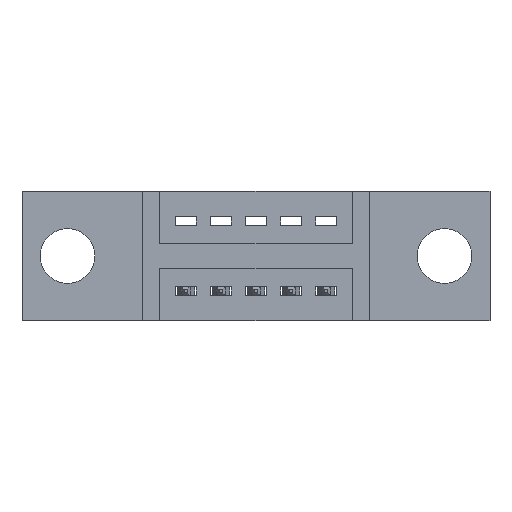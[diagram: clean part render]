
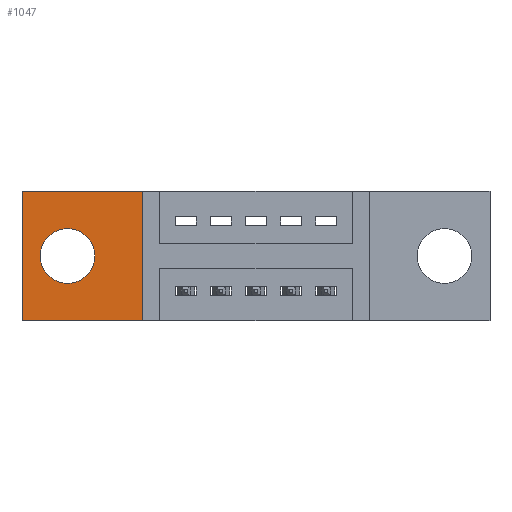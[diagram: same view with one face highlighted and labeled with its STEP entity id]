
A CAD part, front view. The second image highlights one B-rep face of the part: STEP entity #1047.
In plain terms, the highlighted planar face has unit normal (0, -1, 0).
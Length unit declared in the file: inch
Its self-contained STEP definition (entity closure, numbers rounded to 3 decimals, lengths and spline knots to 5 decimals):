
#257 = CIRCLE ( 'NONE', #2262, 0.078 ) ;
#276 = EDGE_CURVE ( 'NONE', #4539, #8290, #7771, .T. ) ;
#394 = VERTEX_POINT ( 'NONE', #4580 ) ;
#573 = FACE_OUTER_BOUND ( 'NONE', #2553, .T. ) ;
#941 = DIRECTION ( 'NONE',  ( -1., 0., 0. ) ) ;
#957 = EDGE_CURVE ( 'NONE', #4929, #394, #257, .T. ) ;
#1047 = ADVANCED_FACE ( 'NONE', ( #6899, #573 ), #6828, .T. ) ;
#1306 = CARTESIAN_POINT ( 'NONE',  ( 0.13, 0.17, -0.185 ) ) ;
#1385 = DIRECTION ( 'NONE',  ( 0., 0., 1. ) ) ;
#1405 = CARTESIAN_POINT ( 'NONE',  ( 0., 0.17, -0.37 ) ) ;
#1478 = CARTESIAN_POINT ( 'NONE',  ( 0., 0.17, 0. ) ) ;
#1729 = DIRECTION ( 'NONE',  ( 1., 0., 0. ) ) ;
#1828 = VERTEX_POINT ( 'NONE', #8216 ) ;
#1973 = CARTESIAN_POINT ( 'NONE',  ( 0., 0.17, 0. ) ) ;
#2034 = DIRECTION ( 'NONE',  ( 0., -1., 0. ) ) ;
#2063 = AXIS2_PLACEMENT_3D ( 'NONE', #1306, #2034, #6825 ) ;
#2262 = AXIS2_PLACEMENT_3D ( 'NONE', #8084, #2614, #6683 ) ;
#2553 = EDGE_LOOP ( 'NONE', ( #7649, #8466, #8158, #4340 ) ) ;
#2614 = DIRECTION ( 'NONE',  ( 0., -1., 0. ) ) ;
#2846 = AXIS2_PLACEMENT_3D ( 'NONE', #1405, #3360, #5383 ) ;
#3050 = CARTESIAN_POINT ( 'NONE',  ( 0., 0.17, -0.37 ) ) ;
#3360 = DIRECTION ( 'NONE',  ( 0., -1., 0. ) ) ;
#3417 = CARTESIAN_POINT ( 'NONE',  ( 0., 0.17, 0. ) ) ;
#4239 = VERTEX_POINT ( 'NONE', #5017 ) ;
#4340 = ORIENTED_EDGE ( 'NONE', *, *, #276, .T. ) ;
#4539 = VERTEX_POINT ( 'NONE', #8808 ) ;
#4580 = CARTESIAN_POINT ( 'NONE',  ( 0.13, 0.17, -0.107 ) ) ;
#4612 = EDGE_CURVE ( 'NONE', #394, #4929, #8253, .T. ) ;
#4929 = VERTEX_POINT ( 'NONE', #8529 ) ;
#4957 = VECTOR ( 'NONE', #1729, 39.37008 ) ;
#5017 = CARTESIAN_POINT ( 'NONE',  ( 0., 0.17, -0.37 ) ) ;
#5274 = LINE ( 'NONE', #5481, #8088 ) ;
#5383 = DIRECTION ( 'NONE',  ( 0., 0., -1. ) ) ;
#5434 = DIRECTION ( 'NONE',  ( 0., 0., -1. ) ) ;
#5479 = LINE ( 'NONE', #1973, #7528 ) ;
#5481 = CARTESIAN_POINT ( 'NONE',  ( 0.3425, 0.17, 0. ) ) ;
#6588 = VECTOR ( 'NONE', #941, 39.37008 ) ;
#6683 = DIRECTION ( 'NONE',  ( 0., 0., -1. ) ) ;
#6819 = ORIENTED_EDGE ( 'NONE', *, *, #4612, .F. ) ;
#6825 = DIRECTION ( 'NONE',  ( 0., 0., -1. ) ) ;
#6828 = PLANE ( 'NONE',  #2846 ) ;
#6867 = EDGE_CURVE ( 'NONE', #4239, #1828, #7106, .T. ) ;
#6899 = FACE_BOUND ( 'NONE', #7347, .T. ) ;
#7106 = LINE ( 'NONE', #3050, #4957 ) ;
#7347 = EDGE_LOOP ( 'NONE', ( #6819, #8788 ) ) ;
#7528 = VECTOR ( 'NONE', #5434, 39.37008 ) ;
#7626 = EDGE_CURVE ( 'NONE', #8290, #4239, #5479, .T. ) ;
#7649 = ORIENTED_EDGE ( 'NONE', *, *, #7626, .T. ) ;
#7771 = LINE ( 'NONE', #3417, #6588 ) ;
#8084 = CARTESIAN_POINT ( 'NONE',  ( 0.13, 0.17, -0.185 ) ) ;
#8088 = VECTOR ( 'NONE', #1385, 39.37008 ) ;
#8158 = ORIENTED_EDGE ( 'NONE', *, *, #8256, .T. ) ;
#8216 = CARTESIAN_POINT ( 'NONE',  ( 0.3425, 0.17, -0.37 ) ) ;
#8253 = CIRCLE ( 'NONE', #2063, 0.078 ) ;
#8256 = EDGE_CURVE ( 'NONE', #1828, #4539, #5274, .T. ) ;
#8290 = VERTEX_POINT ( 'NONE', #1478 ) ;
#8466 = ORIENTED_EDGE ( 'NONE', *, *, #6867, .T. ) ;
#8529 = CARTESIAN_POINT ( 'NONE',  ( 0.13, 0.17, -0.263 ) ) ;
#8788 = ORIENTED_EDGE ( 'NONE', *, *, #957, .F. ) ;
#8808 = CARTESIAN_POINT ( 'NONE',  ( 0.3425, 0.17, 0. ) ) ;
